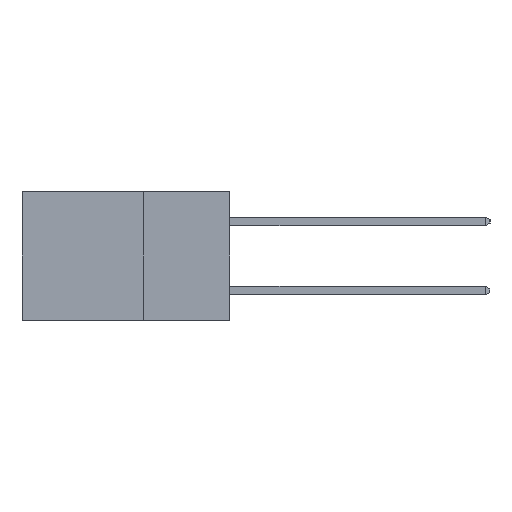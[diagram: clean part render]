
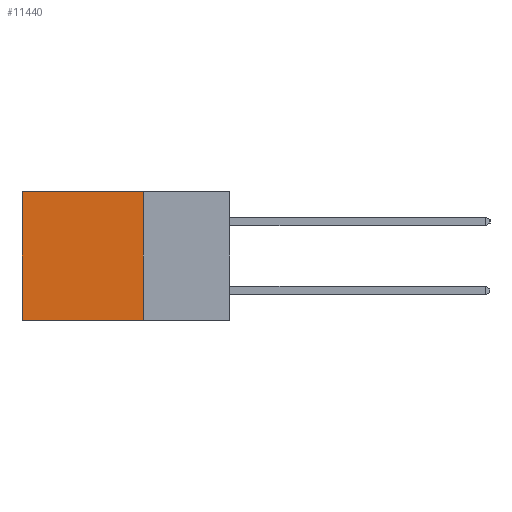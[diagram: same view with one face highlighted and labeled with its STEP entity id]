
A CAD part, left-side view. The second image highlights one B-rep face of the part: STEP entity #11440.
In plain terms, the highlighted planar face has unit normal (-1, 0, 0).
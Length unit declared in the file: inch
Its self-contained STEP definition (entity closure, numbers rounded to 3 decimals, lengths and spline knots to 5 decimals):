
#449 = ORIENTED_EDGE ( 'NONE', *, *, #6686, .F. ) ;
#1071 = CARTESIAN_POINT ( 'NONE',  ( 0.298, 0.25, 0. ) ) ;
#2394 = DIRECTION ( 'NONE',  ( 0., 0., -1. ) ) ;
#2908 = CARTESIAN_POINT ( 'NONE',  ( 0.298, 0.25, 0. ) ) ;
#2963 = CARTESIAN_POINT ( 'NONE',  ( 0.298, 0.25, -0.37 ) ) ;
#3148 = VERTEX_POINT ( 'NONE', #8519 ) ;
#3739 = VECTOR ( 'NONE', #13357, 39.37008 ) ;
#4010 = VERTEX_POINT ( 'NONE', #7048 ) ;
#4282 = ORIENTED_EDGE ( 'NONE', *, *, #13065, .T. ) ;
#5606 = CARTESIAN_POINT ( 'NONE',  ( 0.298, 0.25, 0. ) ) ;
#5823 = CARTESIAN_POINT ( 'NONE',  ( 0.298, 0.6, 0. ) ) ;
#6309 = LINE ( 'NONE', #2963, #3739 ) ;
#6686 = EDGE_CURVE ( 'NONE', #3148, #4010, #6309, .T. ) ;
#7048 = CARTESIAN_POINT ( 'NONE',  ( 0.298, 0.6, -0.37 ) ) ;
#7419 = PLANE ( 'NONE',  #11168 ) ;
#7959 = VERTEX_POINT ( 'NONE', #9713 ) ;
#8415 = VECTOR ( 'NONE', #15267, 39.37008 ) ;
#8519 = CARTESIAN_POINT ( 'NONE',  ( 0.298, 0.25, -0.37 ) ) ;
#8649 = FACE_OUTER_BOUND ( 'NONE', #10837, .T. ) ;
#9713 = CARTESIAN_POINT ( 'NONE',  ( 0.298, 0.6, 0. ) ) ;
#9874 = DIRECTION ( 'NONE',  ( 1., 0., 0. ) ) ;
#10574 = EDGE_CURVE ( 'NONE', #7959, #4010, #11550, .T. ) ;
#10837 = EDGE_LOOP ( 'NONE', ( #13393, #449, #13756, #4282 ) ) ;
#11168 = AXIS2_PLACEMENT_3D ( 'NONE', #1071, #9874, #2394 ) ;
#11440 = ADVANCED_FACE ( 'NONE', ( #8649 ), #7419, .F. ) ;
#11550 = LINE ( 'NONE', #5823, #14444 ) ;
#11838 = VECTOR ( 'NONE', #13077, 39.37008 ) ;
#11991 = DIRECTION ( 'NONE',  ( 0., 0., -1. ) ) ;
#12624 = LINE ( 'NONE', #5606, #11838 ) ;
#13065 = EDGE_CURVE ( 'NONE', #13087, #7959, #14939, .T. ) ;
#13077 = DIRECTION ( 'NONE',  ( 0., 0., -1. ) ) ;
#13087 = VERTEX_POINT ( 'NONE', #2908 ) ;
#13357 = DIRECTION ( 'NONE',  ( 0., 1., 0. ) ) ;
#13393 = ORIENTED_EDGE ( 'NONE', *, *, #10574, .T. ) ;
#13670 = EDGE_CURVE ( 'NONE', #13087, #3148, #12624, .T. ) ;
#13756 = ORIENTED_EDGE ( 'NONE', *, *, #13670, .F. ) ;
#14008 = CARTESIAN_POINT ( 'NONE',  ( 0.298, 0.25, 0. ) ) ;
#14444 = VECTOR ( 'NONE', #11991, 39.37008 ) ;
#14939 = LINE ( 'NONE', #14008, #8415 ) ;
#15267 = DIRECTION ( 'NONE',  ( 0., 1., 0. ) ) ;
